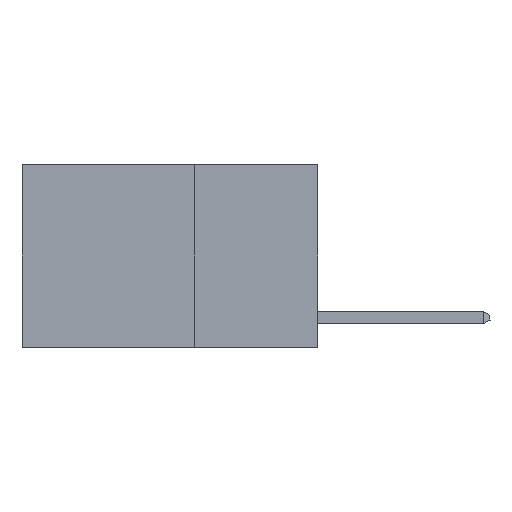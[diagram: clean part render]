
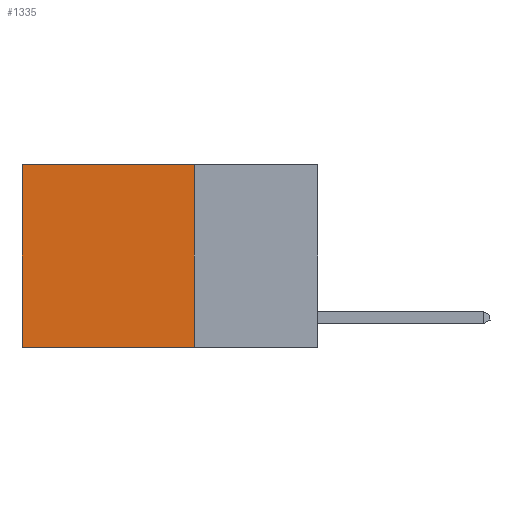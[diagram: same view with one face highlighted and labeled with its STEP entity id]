
A CAD part, left-side view. The second image highlights one B-rep face of the part: STEP entity #1335.
In plain terms, the highlighted planar face has unit normal (-1, 0, 0).
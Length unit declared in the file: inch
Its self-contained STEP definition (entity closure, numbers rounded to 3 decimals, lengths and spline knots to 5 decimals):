
#42 = AXIS2_PLACEMENT_3D ( 'NONE', #3836, #4755, #11064 ) ;
#65 = CARTESIAN_POINT ( 'NONE',  ( 0.2625, 0.25, -0.37 ) ) ;
#637 = ORIENTED_EDGE ( 'NONE', *, *, #9041, .F. ) ;
#1071 = EDGE_LOOP ( 'NONE', ( #6621, #11359, #637, #8484 ) ) ;
#1335 = ADVANCED_FACE ( 'NONE', ( #3038 ), #9226, .F. ) ;
#1618 = DIRECTION ( 'NONE',  ( 0., 0., -1. ) ) ;
#2528 = VECTOR ( 'NONE', #9436, 39.37008 ) ;
#2565 = EDGE_CURVE ( 'NONE', #8845, #3894, #8620, .T. ) ;
#3002 = CARTESIAN_POINT ( 'NONE',  ( 0.2625, 0.6, -0.37 ) ) ;
#3038 = FACE_OUTER_BOUND ( 'NONE', #1071, .T. ) ;
#3139 = CARTESIAN_POINT ( 'NONE',  ( 0.2625, 0.25, 0. ) ) ;
#3836 = CARTESIAN_POINT ( 'NONE',  ( 0.2625, 0.25, 0. ) ) ;
#3859 = VECTOR ( 'NONE', #9071, 39.37008 ) ;
#3894 = VERTEX_POINT ( 'NONE', #3002 ) ;
#4265 = CARTESIAN_POINT ( 'NONE',  ( 0.2625, 0.25, 0. ) ) ;
#4622 = VECTOR ( 'NONE', #1618, 39.37008 ) ;
#4755 = DIRECTION ( 'NONE',  ( 1., 0., 0. ) ) ;
#4898 = CARTESIAN_POINT ( 'NONE',  ( 0.2625, 0.25, -0.37 ) ) ;
#4941 = LINE ( 'NONE', #3139, #2528 ) ;
#5235 = CARTESIAN_POINT ( 'NONE',  ( 0.2625, 0.6, 0. ) ) ;
#6621 = ORIENTED_EDGE ( 'NONE', *, *, #7846, .T. ) ;
#6704 = LINE ( 'NONE', #4265, #8512 ) ;
#6975 = EDGE_CURVE ( 'NONE', #7208, #10277, #4941, .T. ) ;
#7208 = VERTEX_POINT ( 'NONE', #10674 ) ;
#7846 = EDGE_CURVE ( 'NONE', #10277, #3894, #9675, .T. ) ;
#8484 = ORIENTED_EDGE ( 'NONE', *, *, #6975, .T. ) ;
#8512 = VECTOR ( 'NONE', #9643, 39.37008 ) ;
#8620 = LINE ( 'NONE', #65, #3859 ) ;
#8845 = VERTEX_POINT ( 'NONE', #4898 ) ;
#9041 = EDGE_CURVE ( 'NONE', #7208, #8845, #6704, .T. ) ;
#9071 = DIRECTION ( 'NONE',  ( 0., 1., 0. ) ) ;
#9226 = PLANE ( 'NONE',  #42 ) ;
#9436 = DIRECTION ( 'NONE',  ( 0., 1., 0. ) ) ;
#9643 = DIRECTION ( 'NONE',  ( 0., 0., -1. ) ) ;
#9675 = LINE ( 'NONE', #5235, #4622 ) ;
#10277 = VERTEX_POINT ( 'NONE', #10425 ) ;
#10425 = CARTESIAN_POINT ( 'NONE',  ( 0.2625, 0.6, 0. ) ) ;
#10674 = CARTESIAN_POINT ( 'NONE',  ( 0.2625, 0.25, 0. ) ) ;
#11064 = DIRECTION ( 'NONE',  ( 0., 0., -1. ) ) ;
#11359 = ORIENTED_EDGE ( 'NONE', *, *, #2565, .F. ) ;
